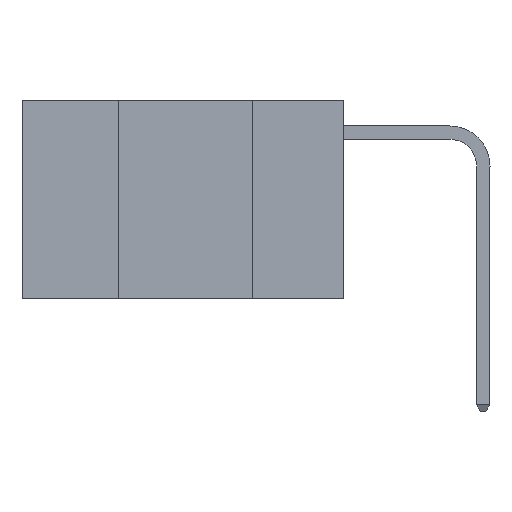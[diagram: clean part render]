
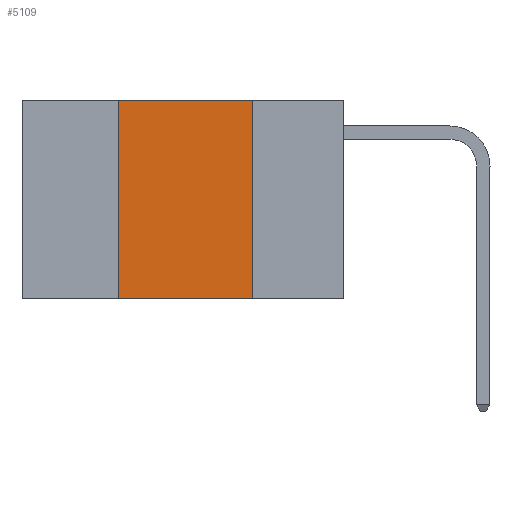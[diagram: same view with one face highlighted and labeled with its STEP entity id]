
A CAD part, left-side view. The second image highlights one B-rep face of the part: STEP entity #5109.
In plain terms, the highlighted planar face has unit normal (-1, 0, 0).
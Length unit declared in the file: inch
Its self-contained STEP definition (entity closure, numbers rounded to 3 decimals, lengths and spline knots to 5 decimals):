
#12 = DIRECTION ( 'NONE',  ( 0., 0., -1. ) ) ;
#140 = CARTESIAN_POINT ( 'NONE',  ( 0., 0.42, 0. ) ) ;
#678 = LINE ( 'NONE', #723, #3524 ) ;
#723 = CARTESIAN_POINT ( 'NONE',  ( 0., 0.42, 0. ) ) ;
#770 = LINE ( 'NONE', #13055, #6048 ) ;
#1864 = DIRECTION ( 'NONE',  ( 0., 0., -1. ) ) ;
#1913 = EDGE_CURVE ( 'NONE', #6465, #10100, #7064, .T. ) ;
#2243 = CARTESIAN_POINT ( 'NONE',  ( 0., 0.6, -0.37 ) ) ;
#3515 = VECTOR ( 'NONE', #1864, 39.37008 ) ;
#3524 = VECTOR ( 'NONE', #12425, 39.37008 ) ;
#3626 = CARTESIAN_POINT ( 'NONE',  ( 0., 0.6, 0. ) ) ;
#4856 = CARTESIAN_POINT ( 'NONE',  ( 0., 0.17, 0. ) ) ;
#5109 = ADVANCED_FACE ( 'NONE', ( #11236 ), #14013, .F. ) ;
#5180 = EDGE_CURVE ( 'NONE', #6423, #6465, #770, .T. ) ;
#6048 = VECTOR ( 'NONE', #14212, 39.37008 ) ;
#6423 = VERTEX_POINT ( 'NONE', #140 ) ;
#6465 = VERTEX_POINT ( 'NONE', #8565 ) ;
#6871 = ORIENTED_EDGE ( 'NONE', *, *, #8080, .F. ) ;
#7064 = LINE ( 'NONE', #4856, #3515 ) ;
#7225 = DIRECTION ( 'NONE',  ( 1., 0., 0. ) ) ;
#7756 = ORIENTED_EDGE ( 'NONE', *, *, #8217, .T. ) ;
#8080 = EDGE_CURVE ( 'NONE', #8919, #6423, #678, .T. ) ;
#8217 = EDGE_CURVE ( 'NONE', #8919, #10100, #10587, .T. ) ;
#8565 = CARTESIAN_POINT ( 'NONE',  ( 0., 0.17, 0. ) ) ;
#8919 = VERTEX_POINT ( 'NONE', #9581 ) ;
#9581 = CARTESIAN_POINT ( 'NONE',  ( 0., 0.42, -0.37 ) ) ;
#10025 = AXIS2_PLACEMENT_3D ( 'NONE', #3626, #7225, #12 ) ;
#10100 = VERTEX_POINT ( 'NONE', #13703 ) ;
#10587 = LINE ( 'NONE', #2243, #13642 ) ;
#11236 = FACE_OUTER_BOUND ( 'NONE', #14260, .T. ) ;
#11539 = DIRECTION ( 'NONE',  ( 0., -1., 0. ) ) ;
#11676 = ORIENTED_EDGE ( 'NONE', *, *, #1913, .F. ) ;
#12425 = DIRECTION ( 'NONE',  ( 0., 0., 1. ) ) ;
#13055 = CARTESIAN_POINT ( 'NONE',  ( 0., 0.6, 0. ) ) ;
#13642 = VECTOR ( 'NONE', #11539, 39.37008 ) ;
#13703 = CARTESIAN_POINT ( 'NONE',  ( 0., 0.17, -0.37 ) ) ;
#14013 = PLANE ( 'NONE',  #10025 ) ;
#14212 = DIRECTION ( 'NONE',  ( 0., -1., 0. ) ) ;
#14260 = EDGE_LOOP ( 'NONE', ( #11676, #14886, #6871, #7756 ) ) ;
#14886 = ORIENTED_EDGE ( 'NONE', *, *, #5180, .F. ) ;
